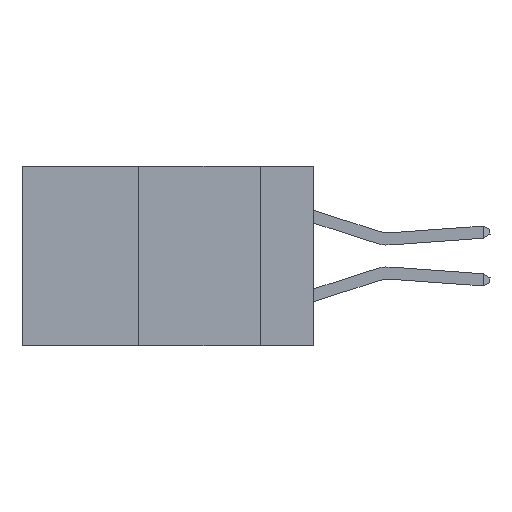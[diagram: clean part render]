
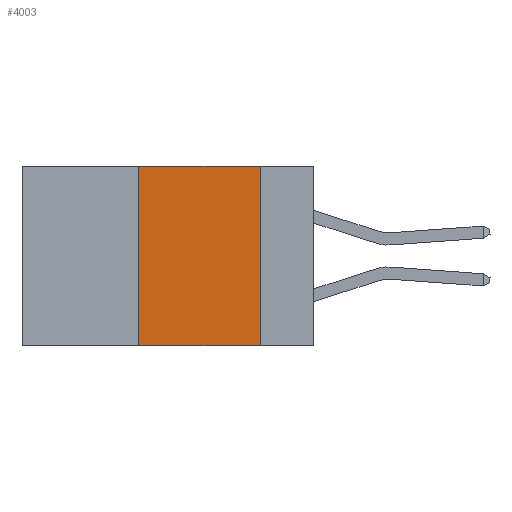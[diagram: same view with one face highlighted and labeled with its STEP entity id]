
A CAD part, left-side view. The second image highlights one B-rep face of the part: STEP entity #4003.
In plain terms, the highlighted planar face has unit normal (-1, 0, 0).
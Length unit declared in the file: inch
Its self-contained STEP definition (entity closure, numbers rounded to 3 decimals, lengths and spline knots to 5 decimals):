
#1259 = DIRECTION ( 'NONE',  ( 0., -1., 0. ) ) ;
#2235 = DIRECTION ( 'NONE',  ( 1., 0., 0. ) ) ;
#2693 = CARTESIAN_POINT ( 'NONE',  ( 0., 0.36, 0. ) ) ;
#3516 = VERTEX_POINT ( 'NONE', #26348 ) ;
#3931 = VERTEX_POINT ( 'NONE', #13838 ) ;
#4003 = ADVANCED_FACE ( 'NONE', ( #34610 ), #19682, .F. ) ;
#4906 = VECTOR ( 'NONE', #1259, 39.37008 ) ;
#5733 = LINE ( 'NONE', #9918, #9745 ) ;
#6093 = EDGE_LOOP ( 'NONE', ( #34998, #6591, #11820, #34250 ) ) ;
#6591 = ORIENTED_EDGE ( 'NONE', *, *, #10131, .F. ) ;
#7787 = EDGE_CURVE ( 'NONE', #18452, #3516, #13371, .T. ) ;
#8468 = CARTESIAN_POINT ( 'NONE',  ( 0., 0.36, -0.37 ) ) ;
#9745 = VECTOR ( 'NONE', #12533, 39.37008 ) ;
#9918 = CARTESIAN_POINT ( 'NONE',  ( 0., 0.11, 0. ) ) ;
#10131 = EDGE_CURVE ( 'NONE', #3931, #28141, #16312, .T. ) ;
#11243 = CARTESIAN_POINT ( 'NONE',  ( 0., 0.6, 0. ) ) ;
#11820 = ORIENTED_EDGE ( 'NONE', *, *, #16912, .F. ) ;
#12533 = DIRECTION ( 'NONE',  ( 0., 0., -1. ) ) ;
#13371 = LINE ( 'NONE', #35450, #4906 ) ;
#13634 = VECTOR ( 'NONE', #28928, 39.37008 ) ;
#13838 = CARTESIAN_POINT ( 'NONE',  ( 0., 0.36, 0. ) ) ;
#13910 = DIRECTION ( 'NONE',  ( 0., 0., 1. ) ) ;
#16312 = LINE ( 'NONE', #26292, #13634 ) ;
#16503 = AXIS2_PLACEMENT_3D ( 'NONE', #11243, #2235, #30837 ) ;
#16865 = LINE ( 'NONE', #2693, #28959 ) ;
#16912 = EDGE_CURVE ( 'NONE', #18452, #3931, #16865, .T. ) ;
#17181 = EDGE_CURVE ( 'NONE', #28141, #3516, #5733, .T. ) ;
#17268 = CARTESIAN_POINT ( 'NONE',  ( 0., 0.11, 0. ) ) ;
#18452 = VERTEX_POINT ( 'NONE', #8468 ) ;
#19682 = PLANE ( 'NONE',  #16503 ) ;
#26292 = CARTESIAN_POINT ( 'NONE',  ( 0., 0.6, 0. ) ) ;
#26348 = CARTESIAN_POINT ( 'NONE',  ( 0., 0.11, -0.37 ) ) ;
#28141 = VERTEX_POINT ( 'NONE', #17268 ) ;
#28928 = DIRECTION ( 'NONE',  ( 0., -1., 0. ) ) ;
#28959 = VECTOR ( 'NONE', #13910, 39.37008 ) ;
#30837 = DIRECTION ( 'NONE',  ( 0., 0., -1. ) ) ;
#34250 = ORIENTED_EDGE ( 'NONE', *, *, #7787, .T. ) ;
#34610 = FACE_OUTER_BOUND ( 'NONE', #6093, .T. ) ;
#34998 = ORIENTED_EDGE ( 'NONE', *, *, #17181, .F. ) ;
#35450 = CARTESIAN_POINT ( 'NONE',  ( 0., 0.6, -0.37 ) ) ;
